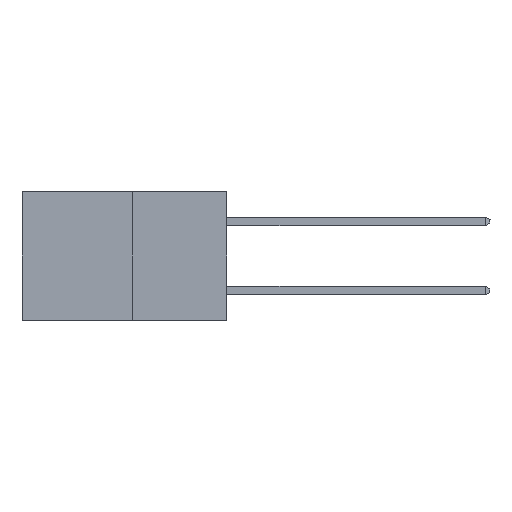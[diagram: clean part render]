
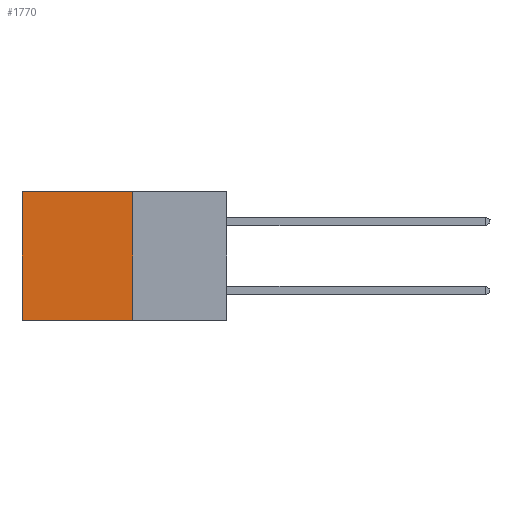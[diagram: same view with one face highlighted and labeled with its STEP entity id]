
A CAD part, left-side view. The second image highlights one B-rep face of the part: STEP entity #1770.
In plain terms, the highlighted planar face has unit normal (-1, 0, 0).
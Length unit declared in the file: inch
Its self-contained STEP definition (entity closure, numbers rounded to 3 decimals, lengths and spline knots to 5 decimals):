
#93 = CARTESIAN_POINT ( 'NONE',  ( 0.277, 0.59, -0.37 ) ) ;
#568 = AXIS2_PLACEMENT_3D ( 'NONE', #7210, #7283, #5054 ) ;
#772 = CARTESIAN_POINT ( 'NONE',  ( 0.277, 0.27, 0. ) ) ;
#1115 = CARTESIAN_POINT ( 'NONE',  ( 0.277, 0.27, 0. ) ) ;
#1344 = PLANE ( 'NONE',  #568 ) ;
#1451 = VECTOR ( 'NONE', #2983, 39.37008 ) ;
#1643 = LINE ( 'NONE', #5609, #5240 ) ;
#1770 = ADVANCED_FACE ( 'NONE', ( #4030 ), #1344, .F. ) ;
#1863 = DIRECTION ( 'NONE',  ( 0., 0., -1. ) ) ;
#2161 = EDGE_CURVE ( 'NONE', #4727, #8202, #7420, .T. ) ;
#2268 = VERTEX_POINT ( 'NONE', #4001 ) ;
#2573 = EDGE_CURVE ( 'NONE', #4727, #2268, #8571, .T. ) ;
#2938 = ORIENTED_EDGE ( 'NONE', *, *, #4396, .F. ) ;
#2983 = DIRECTION ( 'NONE',  ( 0., 0., -1. ) ) ;
#3702 = CARTESIAN_POINT ( 'NONE',  ( 0.277, 0.27, -0.37 ) ) ;
#4001 = CARTESIAN_POINT ( 'NONE',  ( 0.277, 0.59, 0. ) ) ;
#4030 = FACE_OUTER_BOUND ( 'NONE', #4991, .T. ) ;
#4396 = EDGE_CURVE ( 'NONE', #8202, #9025, #1643, .T. ) ;
#4727 = VERTEX_POINT ( 'NONE', #1115 ) ;
#4991 = EDGE_LOOP ( 'NONE', ( #6567, #2938, #7213, #5513 ) ) ;
#5054 = DIRECTION ( 'NONE',  ( 0., 0., -1. ) ) ;
#5177 = LINE ( 'NONE', #8289, #6895 ) ;
#5240 = VECTOR ( 'NONE', #8423, 39.37008 ) ;
#5513 = ORIENTED_EDGE ( 'NONE', *, *, #2573, .T. ) ;
#5609 = CARTESIAN_POINT ( 'NONE',  ( 0.277, 0.27, -0.37 ) ) ;
#6047 = DIRECTION ( 'NONE',  ( 0., 1., 0. ) ) ;
#6567 = ORIENTED_EDGE ( 'NONE', *, *, #7821, .T. ) ;
#6895 = VECTOR ( 'NONE', #1863, 39.37008 ) ;
#7201 = VECTOR ( 'NONE', #6047, 39.37008 ) ;
#7210 = CARTESIAN_POINT ( 'NONE',  ( 0.277, 0.27, -0.37 ) ) ;
#7213 = ORIENTED_EDGE ( 'NONE', *, *, #2161, .F. ) ;
#7283 = DIRECTION ( 'NONE',  ( 1., 0., 0. ) ) ;
#7420 = LINE ( 'NONE', #3702, #1451 ) ;
#7821 = EDGE_CURVE ( 'NONE', #2268, #9025, #5177, .T. ) ;
#8202 = VERTEX_POINT ( 'NONE', #8691 ) ;
#8289 = CARTESIAN_POINT ( 'NONE',  ( 0.277, 0.59, -0.37 ) ) ;
#8423 = DIRECTION ( 'NONE',  ( 0., 1., 0. ) ) ;
#8571 = LINE ( 'NONE', #772, #7201 ) ;
#8691 = CARTESIAN_POINT ( 'NONE',  ( 0.277, 0.27, -0.37 ) ) ;
#9025 = VERTEX_POINT ( 'NONE', #93 ) ;
